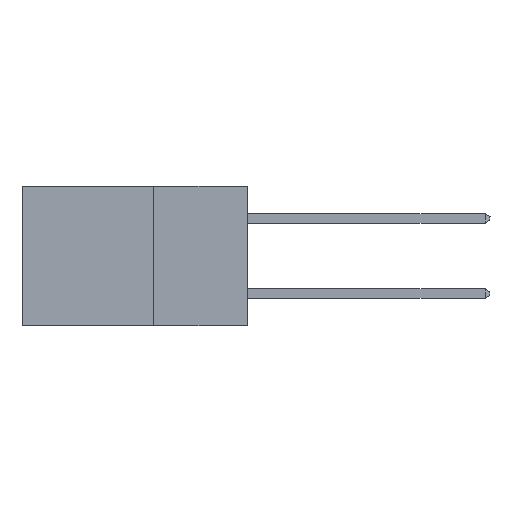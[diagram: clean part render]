
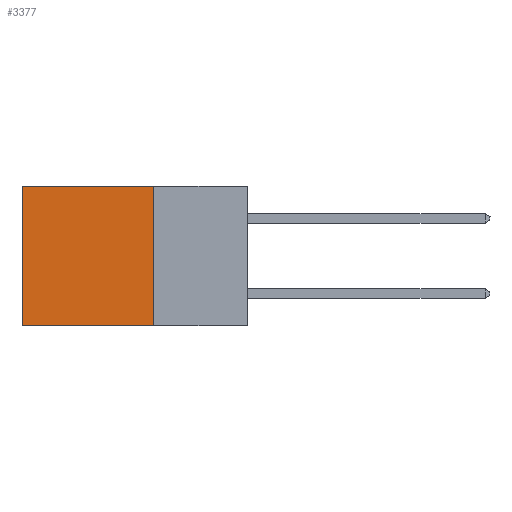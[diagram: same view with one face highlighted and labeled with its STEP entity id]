
A CAD part, left-side view. The second image highlights one B-rep face of the part: STEP entity #3377.
In plain terms, the highlighted planar face has unit normal (-1, 0, 0).
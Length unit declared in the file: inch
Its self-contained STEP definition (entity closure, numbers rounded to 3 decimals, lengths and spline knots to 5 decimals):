
#588 = ORIENTED_EDGE ( 'NONE', *, *, #18253, .F. ) ;
#1469 = VECTOR ( 'NONE', #5973, 39.37008 ) ;
#1629 = CARTESIAN_POINT ( 'NONE',  ( 0.298, 0.6, 0. ) ) ;
#2173 = CARTESIAN_POINT ( 'NONE',  ( 0.298, 0.25, 0. ) ) ;
#2514 = EDGE_CURVE ( 'NONE', #11580, #10689, #18522, .T. ) ;
#2826 = CARTESIAN_POINT ( 'NONE',  ( 0.298, 0.25, -0.37 ) ) ;
#3158 = VECTOR ( 'NONE', #16074, 39.37008 ) ;
#3377 = ADVANCED_FACE ( 'NONE', ( #5858 ), #10981, .F. ) ;
#4436 = CARTESIAN_POINT ( 'NONE',  ( 0.298, 0.25, 0. ) ) ;
#4479 = VERTEX_POINT ( 'NONE', #11401 ) ;
#4552 = EDGE_CURVE ( 'NONE', #11580, #9376, #6271, .T. ) ;
#5027 = DIRECTION ( 'NONE',  ( 1., 0., 0. ) ) ;
#5858 = FACE_OUTER_BOUND ( 'NONE', #13555, .T. ) ;
#5973 = DIRECTION ( 'NONE',  ( 0., 0., -1. ) ) ;
#6271 = LINE ( 'NONE', #4436, #1469 ) ;
#7355 = EDGE_CURVE ( 'NONE', #10689, #4479, #7901, .T. ) ;
#7634 = VECTOR ( 'NONE', #12105, 39.37008 ) ;
#7901 = LINE ( 'NONE', #18716, #12949 ) ;
#8688 = CARTESIAN_POINT ( 'NONE',  ( 0.298, 0.25, 0. ) ) ;
#9376 = VERTEX_POINT ( 'NONE', #13418 ) ;
#9566 = DIRECTION ( 'NONE',  ( 0., 0., -1. ) ) ;
#10689 = VERTEX_POINT ( 'NONE', #1629 ) ;
#10981 = PLANE ( 'NONE',  #15925 ) ;
#11192 = CARTESIAN_POINT ( 'NONE',  ( 0.298, 0.25, 0. ) ) ;
#11314 = LINE ( 'NONE', #2826, #7634 ) ;
#11401 = CARTESIAN_POINT ( 'NONE',  ( 0.298, 0.6, -0.37 ) ) ;
#11580 = VERTEX_POINT ( 'NONE', #11192 ) ;
#12105 = DIRECTION ( 'NONE',  ( 0., 1., 0. ) ) ;
#12870 = DIRECTION ( 'NONE',  ( 0., 0., -1. ) ) ;
#12949 = VECTOR ( 'NONE', #12870, 39.37008 ) ;
#13418 = CARTESIAN_POINT ( 'NONE',  ( 0.298, 0.25, -0.37 ) ) ;
#13555 = EDGE_LOOP ( 'NONE', ( #14078, #588, #17258, #14689 ) ) ;
#14078 = ORIENTED_EDGE ( 'NONE', *, *, #7355, .T. ) ;
#14689 = ORIENTED_EDGE ( 'NONE', *, *, #2514, .T. ) ;
#15925 = AXIS2_PLACEMENT_3D ( 'NONE', #2173, #5027, #9566 ) ;
#16074 = DIRECTION ( 'NONE',  ( 0., 1., 0. ) ) ;
#17258 = ORIENTED_EDGE ( 'NONE', *, *, #4552, .F. ) ;
#18253 = EDGE_CURVE ( 'NONE', #9376, #4479, #11314, .T. ) ;
#18522 = LINE ( 'NONE', #8688, #3158 ) ;
#18716 = CARTESIAN_POINT ( 'NONE',  ( 0.298, 0.6, 0. ) ) ;
